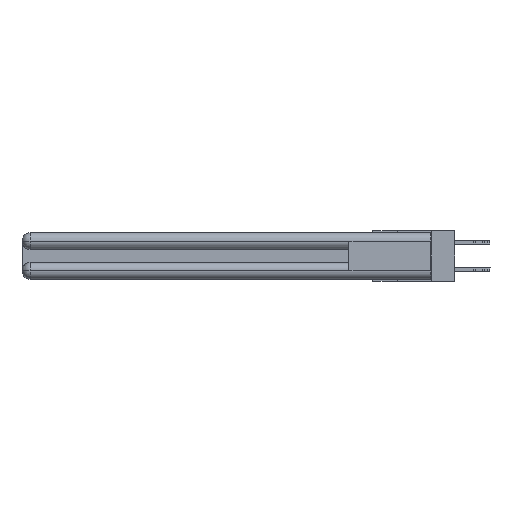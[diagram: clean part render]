
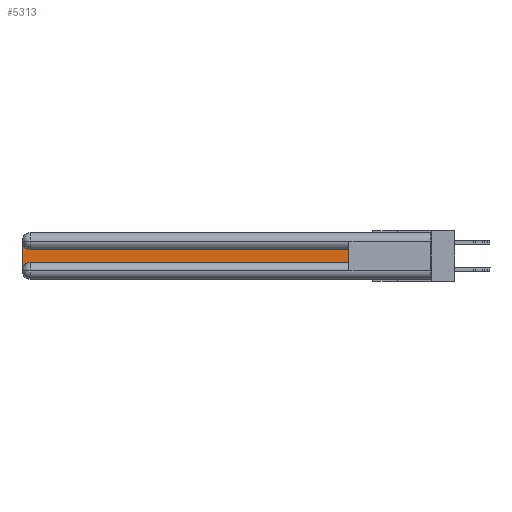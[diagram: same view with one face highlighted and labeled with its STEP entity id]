
A CAD part, left-side view. The second image highlights one B-rep face of the part: STEP entity #5313.
In plain terms, the highlighted planar face has unit normal (-1, 0, 0).
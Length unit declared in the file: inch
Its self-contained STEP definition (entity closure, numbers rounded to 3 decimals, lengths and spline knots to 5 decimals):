
#336 = VERTEX_POINT ( 'NONE', #22207 ) ;
#433 = DIRECTION ( 'NONE',  ( 0., 0., -1. ) ) ;
#1100 = DIRECTION ( 'NONE',  ( 0., -1., 0. ) ) ;
#1256 = DIRECTION ( 'NONE',  ( 1., 0., 0. ) ) ;
#1514 = LINE ( 'NONE', #15255, #25783 ) ;
#2656 = VECTOR ( 'NONE', #1100, 39.37008 ) ;
#2944 = EDGE_LOOP ( 'NONE', ( #22613, #22585, #25244, #9934, #29982, #20363 ) ) ;
#3176 = DIRECTION ( 'NONE',  ( 0., 0., 1. ) ) ;
#3272 = FACE_OUTER_BOUND ( 'NONE', #2944, .T. ) ;
#3306 = EDGE_CURVE ( 'NONE', #9748, #7739, #11376, .T. ) ;
#4122 = CARTESIAN_POINT ( 'NONE',  ( 0.075, 3., -0.0625 ) ) ;
#4312 = DIRECTION ( 'NONE',  ( 0., 0., -1. ) ) ;
#4822 = VERTEX_POINT ( 'NONE', #12436 ) ;
#4937 = CARTESIAN_POINT ( 'NONE',  ( 0.075, 2.94, -0.1225 ) ) ;
#5064 = AXIS2_PLACEMENT_3D ( 'NONE', #20021, #7974, #433 ) ;
#5313 = ADVANCED_FACE ( 'NONE', ( #3272 ), #25407, .F. ) ;
#7739 = VERTEX_POINT ( 'NONE', #12634 ) ;
#7974 = DIRECTION ( 'NONE',  ( 1., 0., 0. ) ) ;
#9180 = AXIS2_PLACEMENT_3D ( 'NONE', #12132, #24426, #26866 ) ;
#9452 = LINE ( 'NONE', #29952, #10551 ) ;
#9748 = VERTEX_POINT ( 'NONE', #25120 ) ;
#9934 = ORIENTED_EDGE ( 'NONE', *, *, #15190, .T. ) ;
#10551 = VECTOR ( 'NONE', #25380, 39.37008 ) ;
#11376 = LINE ( 'NONE', #20334, #12858 ) ;
#12132 = CARTESIAN_POINT ( 'NONE',  ( 0.075, 2.94, -0.2775 ) ) ;
#12436 = CARTESIAN_POINT ( 'NONE',  ( 0.075, 3., -0.2775 ) ) ;
#12634 = CARTESIAN_POINT ( 'NONE',  ( 0.075, 0.6, -0.1225 ) ) ;
#12858 = VECTOR ( 'NONE', #3176, 39.37008 ) ;
#13258 = DIRECTION ( 'NONE',  ( 0., 1., 0. ) ) ;
#14484 = VERTEX_POINT ( 'NONE', #4122 ) ;
#15190 = EDGE_CURVE ( 'NONE', #4822, #336, #28336, .T. ) ;
#15255 = CARTESIAN_POINT ( 'NONE',  ( 0.075, 0.6, -0.1225 ) ) ;
#15531 = LINE ( 'NONE', #15603, #2656 ) ;
#15603 = CARTESIAN_POINT ( 'NONE',  ( 0.075, 0.6, -0.2175 ) ) ;
#15751 = CARTESIAN_POINT ( 'NONE',  ( 0.075, 3., -0.1225 ) ) ;
#17444 = AXIS2_PLACEMENT_3D ( 'NONE', #15751, #1256, #4312 ) ;
#20021 = CARTESIAN_POINT ( 'NONE',  ( 0.075, 2.94, -0.0625 ) ) ;
#20334 = CARTESIAN_POINT ( 'NONE',  ( 0.075, 0.6, -0.2175 ) ) ;
#20363 = ORIENTED_EDGE ( 'NONE', *, *, #3306, .T. ) ;
#20437 = CIRCLE ( 'NONE', #5064, 0.06 ) ;
#20991 = EDGE_CURVE ( 'NONE', #7739, #29685, #1514, .T. ) ;
#22207 = CARTESIAN_POINT ( 'NONE',  ( 0.075, 2.94, -0.2175 ) ) ;
#22585 = ORIENTED_EDGE ( 'NONE', *, *, #28364, .T. ) ;
#22613 = ORIENTED_EDGE ( 'NONE', *, *, #20991, .T. ) ;
#24426 = DIRECTION ( 'NONE',  ( 1., 0., 0. ) ) ;
#25120 = CARTESIAN_POINT ( 'NONE',  ( 0.075, 0.6, -0.2175 ) ) ;
#25244 = ORIENTED_EDGE ( 'NONE', *, *, #29978, .T. ) ;
#25380 = DIRECTION ( 'NONE',  ( 0., 0., -1. ) ) ;
#25407 = PLANE ( 'NONE',  #17444 ) ;
#25783 = VECTOR ( 'NONE', #13258, 39.37008 ) ;
#26866 = DIRECTION ( 'NONE',  ( 0., 0., -1. ) ) ;
#27851 = EDGE_CURVE ( 'NONE', #336, #9748, #15531, .T. ) ;
#28336 = CIRCLE ( 'NONE', #9180, 0.06 ) ;
#28364 = EDGE_CURVE ( 'NONE', #29685, #14484, #20437, .T. ) ;
#29685 = VERTEX_POINT ( 'NONE', #4937 ) ;
#29952 = CARTESIAN_POINT ( 'NONE',  ( 0.075, 3., -0.2175 ) ) ;
#29978 = EDGE_CURVE ( 'NONE', #14484, #4822, #9452, .T. ) ;
#29982 = ORIENTED_EDGE ( 'NONE', *, *, #27851, .T. ) ;
